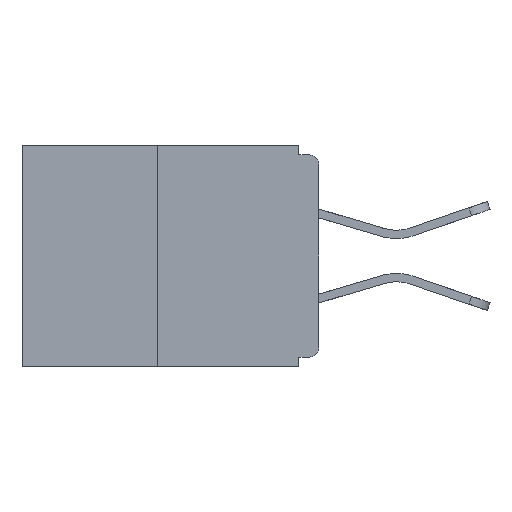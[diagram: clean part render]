
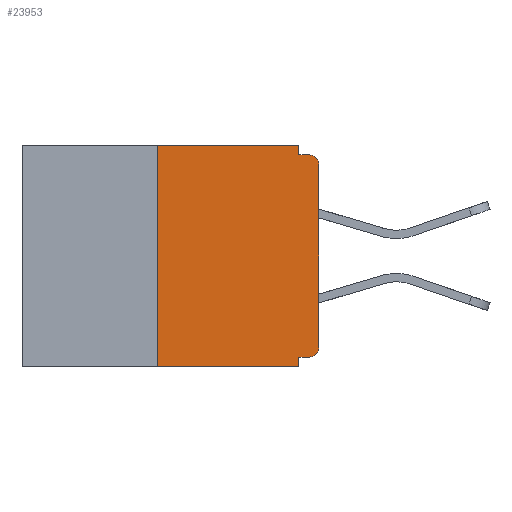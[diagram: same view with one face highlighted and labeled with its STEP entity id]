
A CAD part, left-side view. The second image highlights one B-rep face of the part: STEP entity #23953.
In plain terms, the highlighted planar face has unit normal (-1, 0, 0).
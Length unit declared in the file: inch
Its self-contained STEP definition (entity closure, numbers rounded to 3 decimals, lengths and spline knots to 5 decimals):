
#337 = ORIENTED_EDGE ( 'NONE', *, *, #12519, .F. ) ;
#371 = EDGE_CURVE ( 'NONE', #2739, #11260, #381, .T. ) ;
#381 = LINE ( 'NONE', #1935, #23529 ) ;
#515 = VECTOR ( 'NONE', #8986, 39.37008 ) ;
#815 = CARTESIAN_POINT ( 'NONE',  ( 0., 0.031, -0.015 ) ) ;
#879 = CARTESIAN_POINT ( 'NONE',  ( 0., 0.015, -0.328 ) ) ;
#1324 = VERTEX_POINT ( 'NONE', #28053 ) ;
#1935 = CARTESIAN_POINT ( 'NONE',  ( 0., 0., -0.015 ) ) ;
#2025 = PLANE ( 'NONE',  #25060 ) ;
#2121 = DIRECTION ( 'NONE',  ( 0., -1., 0. ) ) ;
#2242 = CARTESIAN_POINT ( 'NONE',  ( 0., 0.46, -0.343 ) ) ;
#2284 = ORIENTED_EDGE ( 'NONE', *, *, #25847, .T. ) ;
#2739 = VERTEX_POINT ( 'NONE', #815 ) ;
#3257 = ORIENTED_EDGE ( 'NONE', *, *, #371, .F. ) ;
#3440 = EDGE_CURVE ( 'NONE', #15194, #25602, #8100, .T. ) ;
#3567 = VECTOR ( 'NONE', #26260, 39.37008 ) ;
#3733 = CIRCLE ( 'NONE', #18306, 0.015 ) ;
#3982 = ORIENTED_EDGE ( 'NONE', *, *, #3440, .T. ) ;
#4208 = VECTOR ( 'NONE', #20242, 39.37008 ) ;
#4470 = CARTESIAN_POINT ( 'NONE',  ( 0., 0.25, 0. ) ) ;
#4720 = CARTESIAN_POINT ( 'NONE',  ( 0., 0.015, -0.03 ) ) ;
#4724 = VERTEX_POINT ( 'NONE', #8057 ) ;
#4887 = CARTESIAN_POINT ( 'NONE',  ( 0., 0.031, 0. ) ) ;
#4898 = DIRECTION ( 'NONE',  ( 0., 0., -1. ) ) ;
#5686 = EDGE_CURVE ( 'NONE', #4724, #11260, #3733, .T. ) ;
#5836 = ORIENTED_EDGE ( 'NONE', *, *, #22672, .F. ) ;
#5902 = VECTOR ( 'NONE', #4898, 39.37008 ) ;
#6188 = EDGE_CURVE ( 'NONE', #25602, #4724, #13583, .T. ) ;
#6434 = CARTESIAN_POINT ( 'NONE',  ( 0., 0., -0.328 ) ) ;
#6474 = LINE ( 'NONE', #2242, #515 ) ;
#6640 = LINE ( 'NONE', #11783, #5902 ) ;
#6720 = ORIENTED_EDGE ( 'NONE', *, *, #6188, .T. ) ;
#7198 = DIRECTION ( 'NONE',  ( 0., 0., -1. ) ) ;
#7207 = VECTOR ( 'NONE', #7198, 39.37008 ) ;
#7257 = DIRECTION ( 'NONE',  ( 0., 0., -1. ) ) ;
#7662 = FACE_OUTER_BOUND ( 'NONE', #10285, .T. ) ;
#8057 = CARTESIAN_POINT ( 'NONE',  ( 0., 0., -0.03 ) ) ;
#8100 = CIRCLE ( 'NONE', #27419, 0.015 ) ;
#8167 = VERTEX_POINT ( 'NONE', #20660 ) ;
#8986 = DIRECTION ( 'NONE',  ( 0., -1., 0. ) ) ;
#9151 = DIRECTION ( 'NONE',  ( 0., 0., -1. ) ) ;
#9279 = DIRECTION ( 'NONE',  ( -1., 0., 0. ) ) ;
#9366 = CARTESIAN_POINT ( 'NONE',  ( 0., 0.015, -0.313 ) ) ;
#10006 = ORIENTED_EDGE ( 'NONE', *, *, #21181, .F. ) ;
#10285 = EDGE_LOOP ( 'NONE', ( #14008, #337, #2284, #5836, #10006, #3982, #6720, #14916, #3257, #20176 ) ) ;
#11260 = VERTEX_POINT ( 'NONE', #27007 ) ;
#11465 = VECTOR ( 'NONE', #25285, 39.37008 ) ;
#11605 = VERTEX_POINT ( 'NONE', #15404 ) ;
#11783 = CARTESIAN_POINT ( 'NONE',  ( 0., 0.031, -0.343 ) ) ;
#12519 = EDGE_CURVE ( 'NONE', #11605, #24535, #26337, .T. ) ;
#13160 = CARTESIAN_POINT ( 'NONE',  ( 0., 0.46, 0. ) ) ;
#13583 = LINE ( 'NONE', #27423, #11465 ) ;
#13675 = DIRECTION ( 'NONE',  ( -1., 0., 0. ) ) ;
#14008 = ORIENTED_EDGE ( 'NONE', *, *, #27435, .F. ) ;
#14916 = ORIENTED_EDGE ( 'NONE', *, *, #5686, .T. ) ;
#15194 = VERTEX_POINT ( 'NONE', #879 ) ;
#15404 = CARTESIAN_POINT ( 'NONE',  ( 0., 0.25, -0.343 ) ) ;
#15618 = DIRECTION ( 'NONE',  ( 1., 0., 0. ) ) ;
#16336 = VECTOR ( 'NONE', #26302, 39.37008 ) ;
#18306 = AXIS2_PLACEMENT_3D ( 'NONE', #4720, #13675, #7257 ) ;
#18747 = CARTESIAN_POINT ( 'NONE',  ( 0., 0., -0.313 ) ) ;
#18793 = LINE ( 'NONE', #27208, #7207 ) ;
#19280 = VERTEX_POINT ( 'NONE', #4887 ) ;
#20176 = ORIENTED_EDGE ( 'NONE', *, *, #27788, .F. ) ;
#20242 = DIRECTION ( 'NONE',  ( 0., 0., 1. ) ) ;
#20660 = CARTESIAN_POINT ( 'NONE',  ( 0., 0.031, -0.343 ) ) ;
#21181 = EDGE_CURVE ( 'NONE', #15194, #1324, #25315, .T. ) ;
#22276 = CARTESIAN_POINT ( 'NONE',  ( 0., 0.46, 0. ) ) ;
#22316 = LINE ( 'NONE', #13160, #16336 ) ;
#22672 = EDGE_CURVE ( 'NONE', #1324, #8167, #6640, .T. ) ;
#23529 = VECTOR ( 'NONE', #2121, 39.37008 ) ;
#23953 = ADVANCED_FACE ( 'NONE', ( #7662 ), #2025, .F. ) ;
#24535 = VERTEX_POINT ( 'NONE', #27353 ) ;
#25060 = AXIS2_PLACEMENT_3D ( 'NONE', #22276, #15618, #9151 ) ;
#25069 = DIRECTION ( 'NONE',  ( 0., 0., -1. ) ) ;
#25285 = DIRECTION ( 'NONE',  ( 0., 0., 1. ) ) ;
#25315 = LINE ( 'NONE', #6434, #3567 ) ;
#25602 = VERTEX_POINT ( 'NONE', #18747 ) ;
#25847 = EDGE_CURVE ( 'NONE', #11605, #8167, #6474, .T. ) ;
#26260 = DIRECTION ( 'NONE',  ( 0., 1., 0. ) ) ;
#26302 = DIRECTION ( 'NONE',  ( 0., -1., 0. ) ) ;
#26337 = LINE ( 'NONE', #4470, #4208 ) ;
#27007 = CARTESIAN_POINT ( 'NONE',  ( 0., 0.015, -0.015 ) ) ;
#27208 = CARTESIAN_POINT ( 'NONE',  ( 0., 0.031, 0. ) ) ;
#27353 = CARTESIAN_POINT ( 'NONE',  ( 0., 0.25, 0. ) ) ;
#27419 = AXIS2_PLACEMENT_3D ( 'NONE', #9366, #9279, #25069 ) ;
#27423 = CARTESIAN_POINT ( 'NONE',  ( 0., 0., 0. ) ) ;
#27435 = EDGE_CURVE ( 'NONE', #24535, #19280, #22316, .T. ) ;
#27788 = EDGE_CURVE ( 'NONE', #19280, #2739, #18793, .T. ) ;
#28053 = CARTESIAN_POINT ( 'NONE',  ( 0., 0.031, -0.328 ) ) ;
